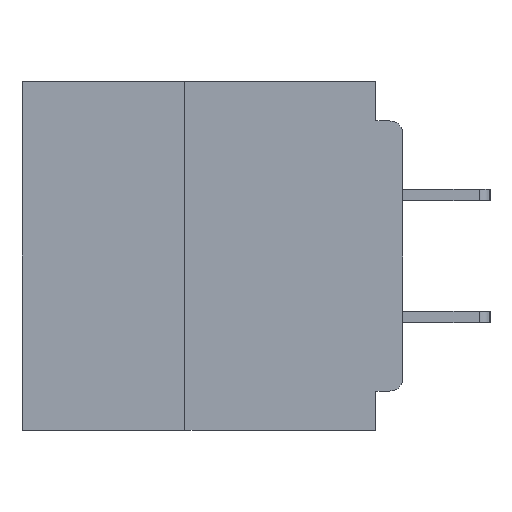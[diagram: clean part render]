
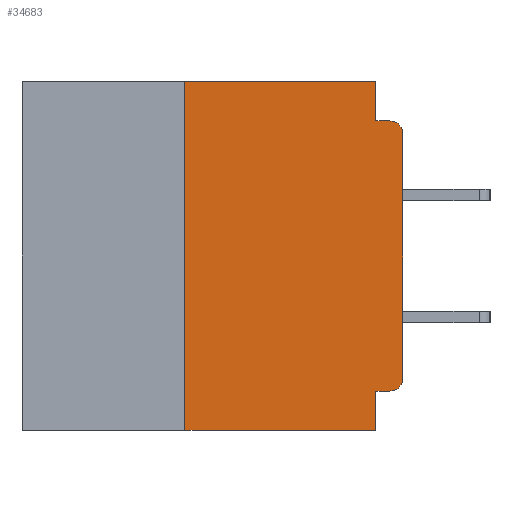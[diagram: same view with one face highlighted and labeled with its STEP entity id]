
A CAD part, left-side view. The second image highlights one B-rep face of the part: STEP entity #34683.
In plain terms, the highlighted planar face has unit normal (-1, 0, 0).
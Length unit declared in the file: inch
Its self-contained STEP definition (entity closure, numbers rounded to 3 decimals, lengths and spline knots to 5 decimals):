
#96 = CARTESIAN_POINT ( 'NONE',  ( 0., 0., 0. ) ) ;
#405 = AXIS2_PLACEMENT_3D ( 'NONE', #5999, #5653, #5525 ) ;
#552 = AXIS2_PLACEMENT_3D ( 'NONE', #3460, #22971, #6242 ) ;
#1384 = LINE ( 'NONE', #11351, #22766 ) ;
#1697 = DIRECTION ( 'NONE',  ( 0., -1., 0. ) ) ;
#1782 = VERTEX_POINT ( 'NONE', #34228 ) ;
#2072 = DIRECTION ( 'NONE',  ( 0., -1., 0. ) ) ;
#2305 = VERTEX_POINT ( 'NONE', #9377 ) ;
#2745 = EDGE_CURVE ( 'NONE', #27105, #2305, #25199, .T. ) ;
#3460 = CARTESIAN_POINT ( 'NONE',  ( 0., 0.015, -0.06 ) ) ;
#3607 = FACE_OUTER_BOUND ( 'NONE', #16773, .T. ) ;
#4085 = EDGE_CURVE ( 'NONE', #19164, #17890, #5892, .T. ) ;
#4151 = ORIENTED_EDGE ( 'NONE', *, *, #5763, .T. ) ;
#4176 = CARTESIAN_POINT ( 'NONE',  ( 0., 0.25, -0.4 ) ) ;
#5525 = DIRECTION ( 'NONE',  ( 0., 0., -1. ) ) ;
#5653 = DIRECTION ( 'NONE',  ( -1., 0., 0. ) ) ;
#5763 = EDGE_CURVE ( 'NONE', #22326, #32345, #14587, .T. ) ;
#5892 = CIRCLE ( 'NONE', #405, 0.015 ) ;
#5999 = CARTESIAN_POINT ( 'NONE',  ( 0., 0.015, -0.34 ) ) ;
#6242 = DIRECTION ( 'NONE',  ( 0., 0., -1. ) ) ;
#6473 = VECTOR ( 'NONE', #1697, 39.37008 ) ;
#7912 = EDGE_CURVE ( 'NONE', #19164, #26072, #11360, .T. ) ;
#9377 = CARTESIAN_POINT ( 'NONE',  ( 0., 0.031, -0.045 ) ) ;
#10789 = EDGE_CURVE ( 'NONE', #2305, #32345, #19297, .T. ) ;
#10913 = ORIENTED_EDGE ( 'NONE', *, *, #19091, .F. ) ;
#11351 = CARTESIAN_POINT ( 'NONE',  ( 0., 0.031, -0.4 ) ) ;
#11360 = LINE ( 'NONE', #19143, #17047 ) ;
#11854 = VECTOR ( 'NONE', #34776, 39.37008 ) ;
#12303 = CARTESIAN_POINT ( 'NONE',  ( 0., 0.031, 0. ) ) ;
#12572 = VERTEX_POINT ( 'NONE', #4176 ) ;
#13261 = ORIENTED_EDGE ( 'NONE', *, *, #10789, .F. ) ;
#13538 = ORIENTED_EDGE ( 'NONE', *, *, #2745, .F. ) ;
#13918 = LINE ( 'NONE', #26742, #6473 ) ;
#14159 = DIRECTION ( 'NONE',  ( 0., 0., -1. ) ) ;
#14364 = LINE ( 'NONE', #27991, #28392 ) ;
#14587 = CIRCLE ( 'NONE', #552, 0.015 ) ;
#15634 = VECTOR ( 'NONE', #2072, 39.37008 ) ;
#16184 = VECTOR ( 'NONE', #33535, 39.37008 ) ;
#16411 = CARTESIAN_POINT ( 'NONE',  ( 0., 0.437, 0. ) ) ;
#16773 = EDGE_LOOP ( 'NONE', ( #33001, #4151, #13261, #13538, #10913, #34024, #31723, #17368, #20250, #34306 ) ) ;
#16957 = EDGE_CURVE ( 'NONE', #17890, #22326, #17064, .T. ) ;
#17047 = VECTOR ( 'NONE', #24768, 39.37008 ) ;
#17064 = LINE ( 'NONE', #96, #16184 ) ;
#17368 = ORIENTED_EDGE ( 'NONE', *, *, #31097, .F. ) ;
#17754 = VECTOR ( 'NONE', #24613, 39.37008 ) ;
#17890 = VERTEX_POINT ( 'NONE', #24323 ) ;
#18080 = CARTESIAN_POINT ( 'NONE',  ( 0., 0., -0.045 ) ) ;
#18140 = CARTESIAN_POINT ( 'NONE',  ( 0., 0.25, 0. ) ) ;
#19091 = EDGE_CURVE ( 'NONE', #33264, #27105, #31377, .T. ) ;
#19143 = CARTESIAN_POINT ( 'NONE',  ( 0., 0., -0.355 ) ) ;
#19164 = VERTEX_POINT ( 'NONE', #27617 ) ;
#19219 = DIRECTION ( 'NONE',  ( 0., 0., -1. ) ) ;
#19297 = LINE ( 'NONE', #18080, #11854 ) ;
#20250 = ORIENTED_EDGE ( 'NONE', *, *, #7912, .F. ) ;
#21225 = CARTESIAN_POINT ( 'NONE',  ( 0., 0.031, -0.355 ) ) ;
#21363 = AXIS2_PLACEMENT_3D ( 'NONE', #16411, #35957, #19219 ) ;
#22324 = DIRECTION ( 'NONE',  ( 0., 0., 1. ) ) ;
#22326 = VERTEX_POINT ( 'NONE', #22623 ) ;
#22623 = CARTESIAN_POINT ( 'NONE',  ( 0., 0., -0.06 ) ) ;
#22766 = VECTOR ( 'NONE', #14159, 39.37008 ) ;
#22971 = DIRECTION ( 'NONE',  ( -1., 0., 0. ) ) ;
#24323 = CARTESIAN_POINT ( 'NONE',  ( 0., 0., -0.34 ) ) ;
#24613 = DIRECTION ( 'NONE',  ( 0., 0., -1. ) ) ;
#24768 = DIRECTION ( 'NONE',  ( 0., 1., 0. ) ) ;
#24787 = CARTESIAN_POINT ( 'NONE',  ( 0., 0.015, -0.045 ) ) ;
#25199 = LINE ( 'NONE', #35335, #17754 ) ;
#26072 = VERTEX_POINT ( 'NONE', #21225 ) ;
#26742 = CARTESIAN_POINT ( 'NONE',  ( 0., 0.437, -0.4 ) ) ;
#27105 = VERTEX_POINT ( 'NONE', #12303 ) ;
#27125 = CARTESIAN_POINT ( 'NONE',  ( 0., 0.437, 0. ) ) ;
#27617 = CARTESIAN_POINT ( 'NONE',  ( 0., 0.015, -0.355 ) ) ;
#27991 = CARTESIAN_POINT ( 'NONE',  ( 0., 0.25, -0.4 ) ) ;
#28392 = VECTOR ( 'NONE', #22324, 39.37008 ) ;
#30374 = PLANE ( 'NONE',  #21363 ) ;
#31097 = EDGE_CURVE ( 'NONE', #26072, #1782, #1384, .T. ) ;
#31377 = LINE ( 'NONE', #27125, #15634 ) ;
#31723 = ORIENTED_EDGE ( 'NONE', *, *, #32686, .T. ) ;
#32345 = VERTEX_POINT ( 'NONE', #24787 ) ;
#32428 = EDGE_CURVE ( 'NONE', #12572, #33264, #14364, .T. ) ;
#32686 = EDGE_CURVE ( 'NONE', #12572, #1782, #13918, .T. ) ;
#33001 = ORIENTED_EDGE ( 'NONE', *, *, #16957, .T. ) ;
#33264 = VERTEX_POINT ( 'NONE', #18140 ) ;
#33535 = DIRECTION ( 'NONE',  ( 0., 0., 1. ) ) ;
#34024 = ORIENTED_EDGE ( 'NONE', *, *, #32428, .F. ) ;
#34228 = CARTESIAN_POINT ( 'NONE',  ( 0., 0.031, -0.4 ) ) ;
#34306 = ORIENTED_EDGE ( 'NONE', *, *, #4085, .T. ) ;
#34683 = ADVANCED_FACE ( 'NONE', ( #3607 ), #30374, .F. ) ;
#34776 = DIRECTION ( 'NONE',  ( 0., -1., 0. ) ) ;
#35335 = CARTESIAN_POINT ( 'NONE',  ( 0., 0.031, 0. ) ) ;
#35957 = DIRECTION ( 'NONE',  ( 1., 0., 0. ) ) ;
